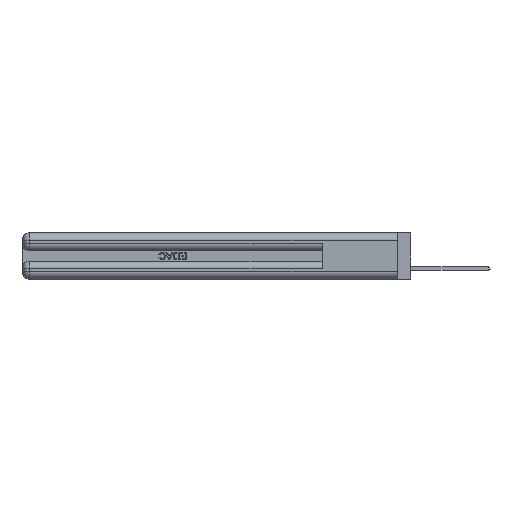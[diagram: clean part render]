
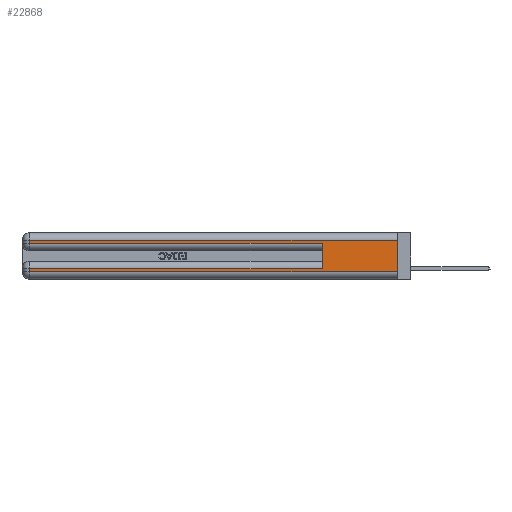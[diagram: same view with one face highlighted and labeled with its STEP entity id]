
A CAD part, left-side view. The second image highlights one B-rep face of the part: STEP entity #22868.
In plain terms, the highlighted planar face has unit normal (-1, 0, 0).
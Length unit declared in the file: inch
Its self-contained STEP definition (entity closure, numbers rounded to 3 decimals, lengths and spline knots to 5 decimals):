
#653 = CARTESIAN_POINT ( 'NONE',  ( 0., 2.94, 0.085 ) ) ;
#1166 = CARTESIAN_POINT ( 'NONE',  ( 0., 2.94, 0.06 ) ) ;
#2864 = DIRECTION ( 'NONE',  ( 0., 0., -1. ) ) ;
#2880 = EDGE_CURVE ( 'NONE', #16925, #38604, #33325, .T. ) ;
#3022 = ORIENTED_EDGE ( 'NONE', *, *, #37238, .T. ) ;
#4103 = EDGE_CURVE ( 'NONE', #20317, #29466, #33123, .T. ) ;
#4218 = CARTESIAN_POINT ( 'NONE',  ( 0., 0., 0.37 ) ) ;
#4235 = CARTESIAN_POINT ( 'NONE',  ( 0., 2.94, 0.37 ) ) ;
#4635 = CARTESIAN_POINT ( 'NONE',  ( 0., 0., 0.06 ) ) ;
#5829 = ORIENTED_EDGE ( 'NONE', *, *, #23614, .T. ) ;
#6446 = CARTESIAN_POINT ( 'NONE',  ( 0., 0.6, 0.145 ) ) ;
#7048 = CARTESIAN_POINT ( 'NONE',  ( 0., 0., 0.285 ) ) ;
#7056 = ORIENTED_EDGE ( 'NONE', *, *, #9258, .T. ) ;
#7937 = VERTEX_POINT ( 'NONE', #20791 ) ;
#8446 = DIRECTION ( 'NONE',  ( 0., -1., 0. ) ) ;
#8448 = ORIENTED_EDGE ( 'NONE', *, *, #20800, .T. ) ;
#9132 = VECTOR ( 'NONE', #2864, 39.37008 ) ;
#9232 = VECTOR ( 'NONE', #18295, 39.37008 ) ;
#9258 = EDGE_CURVE ( 'NONE', #41751, #38604, #18396, .T. ) ;
#9320 = CARTESIAN_POINT ( 'NONE',  ( 0., 0., 0.31 ) ) ;
#9994 = DIRECTION ( 'NONE',  ( 0., 1., 0. ) ) ;
#12196 = FACE_OUTER_BOUND ( 'NONE', #32513, .T. ) ;
#12600 = VECTOR ( 'NONE', #9994, 39.37008 ) ;
#13256 = CARTESIAN_POINT ( 'NONE',  ( 0., 0.6, 0.285 ) ) ;
#15709 = DIRECTION ( 'NONE',  ( 1., 0., 0. ) ) ;
#16925 = VERTEX_POINT ( 'NONE', #21131 ) ;
#17270 = CARTESIAN_POINT ( 'NONE',  ( 0., 0., 0.085 ) ) ;
#17355 = DIRECTION ( 'NONE',  ( 0., 0., 1. ) ) ;
#18295 = DIRECTION ( 'NONE',  ( 0., -1., 0. ) ) ;
#18396 = LINE ( 'NONE', #4635, #30778 ) ;
#18909 = VECTOR ( 'NONE', #45536, 39.37008 ) ;
#19163 = LINE ( 'NONE', #7048, #9232 ) ;
#19486 = DIRECTION ( 'NONE',  ( 0., 0., -1. ) ) ;
#19718 = DIRECTION ( 'NONE',  ( 0., 0., -1. ) ) ;
#20317 = VERTEX_POINT ( 'NONE', #42698 ) ;
#20791 = CARTESIAN_POINT ( 'NONE',  ( 0., 2.94, 0.31 ) ) ;
#20800 = EDGE_CURVE ( 'NONE', #33822, #41751, #28712, .T. ) ;
#21131 = CARTESIAN_POINT ( 'NONE',  ( 0., 0., 0.31 ) ) ;
#22868 = ADVANCED_FACE ( 'NONE', ( #12196 ), #31229, .F. ) ;
#23614 = EDGE_CURVE ( 'NONE', #43557, #29466, #19163, .T. ) ;
#24492 = EDGE_CURVE ( 'NONE', #16925, #7937, #28570, .T. ) ;
#28570 = LINE ( 'NONE', #9320, #12600 ) ;
#28712 = LINE ( 'NONE', #34292, #30434 ) ;
#28878 = DIRECTION ( 'NONE',  ( 0., 1., 0. ) ) ;
#29466 = VERTEX_POINT ( 'NONE', #13256 ) ;
#30434 = VECTOR ( 'NONE', #19718, 39.37008 ) ;
#30778 = VECTOR ( 'NONE', #8446, 39.37008 ) ;
#31229 = PLANE ( 'NONE',  #48271 ) ;
#32513 = EDGE_LOOP ( 'NONE', ( #37154, #47113, #3022, #5829, #33162, #45174, #8448, #7056 ) ) ;
#33123 = LINE ( 'NONE', #6446, #34841 ) ;
#33162 = ORIENTED_EDGE ( 'NONE', *, *, #4103, .F. ) ;
#33325 = LINE ( 'NONE', #40348, #9132 ) ;
#33750 = LINE ( 'NONE', #4235, #18909 ) ;
#33822 = VERTEX_POINT ( 'NONE', #653 ) ;
#34292 = CARTESIAN_POINT ( 'NONE',  ( 0., 2.94, 0.37 ) ) ;
#34841 = VECTOR ( 'NONE', #17355, 39.37008 ) ;
#35128 = EDGE_CURVE ( 'NONE', #20317, #33822, #38554, .T. ) ;
#37154 = ORIENTED_EDGE ( 'NONE', *, *, #2880, .F. ) ;
#37238 = EDGE_CURVE ( 'NONE', #7937, #43557, #33750, .T. ) ;
#38554 = LINE ( 'NONE', #17270, #48601 ) ;
#38604 = VERTEX_POINT ( 'NONE', #48069 ) ;
#40348 = CARTESIAN_POINT ( 'NONE',  ( 0., 0., 0.37 ) ) ;
#41751 = VERTEX_POINT ( 'NONE', #1166 ) ;
#42698 = CARTESIAN_POINT ( 'NONE',  ( 0., 0.6, 0.085 ) ) ;
#43557 = VERTEX_POINT ( 'NONE', #48184 ) ;
#45174 = ORIENTED_EDGE ( 'NONE', *, *, #35128, .T. ) ;
#45536 = DIRECTION ( 'NONE',  ( 0., 0., -1. ) ) ;
#47113 = ORIENTED_EDGE ( 'NONE', *, *, #24492, .T. ) ;
#48069 = CARTESIAN_POINT ( 'NONE',  ( 0., 0., 0.06 ) ) ;
#48184 = CARTESIAN_POINT ( 'NONE',  ( 0., 2.94, 0.285 ) ) ;
#48271 = AXIS2_PLACEMENT_3D ( 'NONE', #4218, #15709, #19486 ) ;
#48601 = VECTOR ( 'NONE', #28878, 39.37008 ) ;
